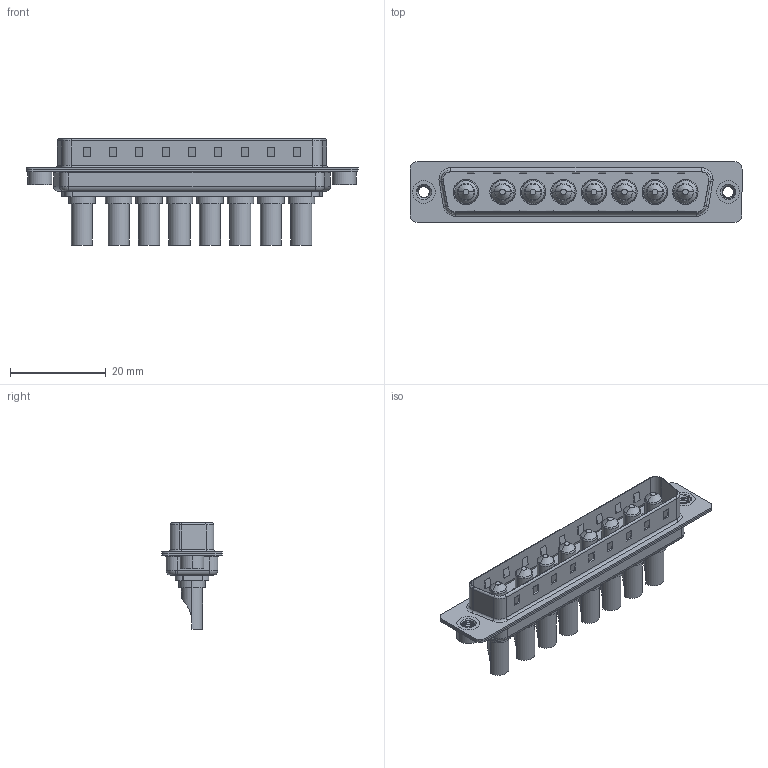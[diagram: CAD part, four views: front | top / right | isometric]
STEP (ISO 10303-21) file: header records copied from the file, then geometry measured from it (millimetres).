
FILE_DESCRIPTION (( 'STEP AP203' ), '1' );
FILE_NAME ('627-8W8-622-3NA.STEP', '2019-05-28T04:41:15', ( '' ), ( '' ), 'SwSTEP 2.0', 'SolidWorks 2016', '' );
FILE_SCHEMA (( 'CONFIG_CONTROL_DESIGN' ));
Length unit declared in the file: millimetre
Products named in the file (7): 627Combo Shell Front_37 Contacts; 627Combo Threaded Rivet_2; 627Combo Shell Rear_37 Contacts; 627-8W8-622-3NA; 627Combo Housing_8W8; Power Pin_30A SC; 627Combo Threaded Rivet_A
Assembly tree (13 placements, depth 2):
  627-8W8-622-3NA
    627Combo Housing_8W8
    627Combo Shell Rear_37 Contacts
    627Combo Shell Front_37 Contacts
    627Combo Threaded Rivet_A
    Power Pin_30A SC  x8
    627Combo Threaded Rivet_2
Bounding box: 69.3 x 12.6 x 22.3 mm (x, y, z)
Volume: 4523.2 mm3; surface area: 10090 mm2
Topology: 21 solids, 21 shells, 779 faces, 1870 edges, 1152 vertices
Faces by surface type: cylinder 318, plane 307, torus 66, cone 66, bspline 22
Entity records: 18959 total; most frequent: CARTESIAN_POINT 5978, DIRECTION 2578, ORIENTED_EDGE 2472, EDGE_CURVE 1236, AXIS2_PLACEMENT_3D 929, VERTEX_POINT 781, LINE 720, VECTOR 720
